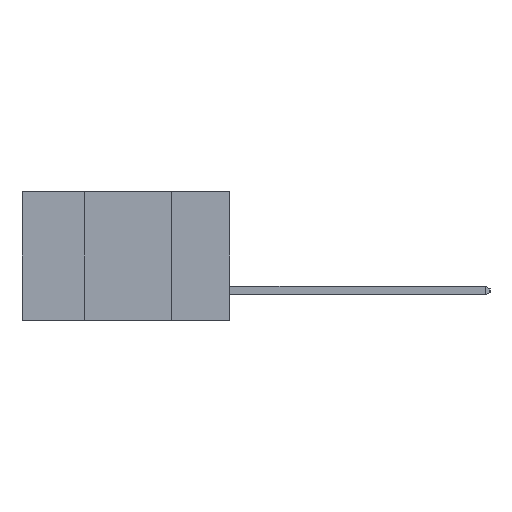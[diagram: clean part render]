
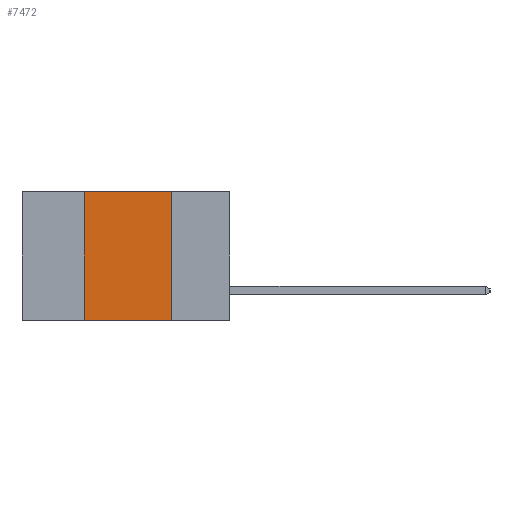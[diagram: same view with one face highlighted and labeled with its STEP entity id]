
A CAD part, left-side view. The second image highlights one B-rep face of the part: STEP entity #7472.
In plain terms, the highlighted planar face has unit normal (-1, 0, 0).
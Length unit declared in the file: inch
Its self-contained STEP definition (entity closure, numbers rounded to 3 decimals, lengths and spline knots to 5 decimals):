
#1752 = VECTOR ( 'NONE', #12428, 39.37008 ) ;
#2313 = LINE ( 'NONE', #12207, #1752 ) ;
#2483 = DIRECTION ( 'NONE',  ( 0., 0., -1. ) ) ;
#2552 = DIRECTION ( 'NONE',  ( 1., 0., 0. ) ) ;
#2583 = CARTESIAN_POINT ( 'NONE',  ( 0., 0.6, 0. ) ) ;
#2630 = PLANE ( 'NONE',  #17694 ) ;
#4445 = EDGE_CURVE ( 'NONE', #10283, #6327, #14483, .T. ) ;
#4709 = ORIENTED_EDGE ( 'NONE', *, *, #10456, .T. ) ;
#4905 = ORIENTED_EDGE ( 'NONE', *, *, #5646, .F. ) ;
#4920 = LINE ( 'NONE', #17280, #14481 ) ;
#5077 = ORIENTED_EDGE ( 'NONE', *, *, #4445, .F. ) ;
#5116 = ORIENTED_EDGE ( 'NONE', *, *, #20286, .F. ) ;
#5646 = EDGE_CURVE ( 'NONE', #19733, #10283, #2313, .T. ) ;
#6311 = CARTESIAN_POINT ( 'NONE',  ( 0., 0.17, -0.37 ) ) ;
#6327 = VERTEX_POINT ( 'NONE', #17207 ) ;
#6686 = DIRECTION ( 'NONE',  ( 0., -1., 0. ) ) ;
#6970 = CARTESIAN_POINT ( 'NONE',  ( 0., 0.6, 0. ) ) ;
#7472 = ADVANCED_FACE ( 'NONE', ( #9860 ), #2630, .F. ) ;
#9451 = VECTOR ( 'NONE', #13712, 39.37008 ) ;
#9860 = FACE_OUTER_BOUND ( 'NONE', #16605, .T. ) ;
#9944 = VERTEX_POINT ( 'NONE', #6311 ) ;
#10022 = LINE ( 'NONE', #11897, #9451 ) ;
#10283 = VERTEX_POINT ( 'NONE', #19942 ) ;
#10456 = EDGE_CURVE ( 'NONE', #19733, #9944, #4920, .T. ) ;
#11897 = CARTESIAN_POINT ( 'NONE',  ( 0., 0.17, -0.37 ) ) ;
#12207 = CARTESIAN_POINT ( 'NONE',  ( 0., 0.42, -0.37 ) ) ;
#12428 = DIRECTION ( 'NONE',  ( 0., 0., 1. ) ) ;
#13712 = DIRECTION ( 'NONE',  ( 0., 0., -1. ) ) ;
#14481 = VECTOR ( 'NONE', #17904, 39.37008 ) ;
#14483 = LINE ( 'NONE', #6970, #19107 ) ;
#15682 = CARTESIAN_POINT ( 'NONE',  ( 0., 0.42, -0.37 ) ) ;
#16605 = EDGE_LOOP ( 'NONE', ( #5116, #5077, #4905, #4709 ) ) ;
#17207 = CARTESIAN_POINT ( 'NONE',  ( 0., 0.17, 0. ) ) ;
#17280 = CARTESIAN_POINT ( 'NONE',  ( 0., 0.6, -0.37 ) ) ;
#17694 = AXIS2_PLACEMENT_3D ( 'NONE', #2583, #2552, #2483 ) ;
#17904 = DIRECTION ( 'NONE',  ( 0., -1., 0. ) ) ;
#19107 = VECTOR ( 'NONE', #6686, 39.37008 ) ;
#19733 = VERTEX_POINT ( 'NONE', #15682 ) ;
#19942 = CARTESIAN_POINT ( 'NONE',  ( 0., 0.42, 0. ) ) ;
#20286 = EDGE_CURVE ( 'NONE', #6327, #9944, #10022, .T. ) ;
